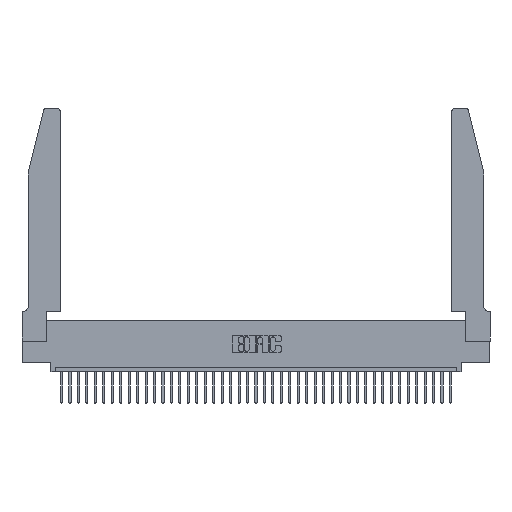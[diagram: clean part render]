
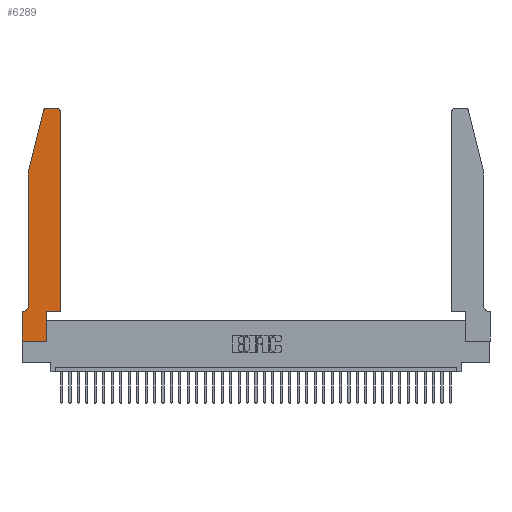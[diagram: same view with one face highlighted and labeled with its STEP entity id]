
A CAD part, top view. The second image highlights one B-rep face of the part: STEP entity #6289.
In plain terms, the highlighted planar face has unit normal (0, 0, 1).
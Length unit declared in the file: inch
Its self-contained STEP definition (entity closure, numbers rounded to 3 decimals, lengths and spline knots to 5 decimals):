
#177 = VECTOR ( 'NONE', #949, 39.37008 ) ;
#435 = CARTESIAN_POINT ( 'NONE',  ( 0.4205, 2.72, 0.37 ) ) ;
#949 = DIRECTION ( 'NONE',  ( -0.239, -0.971, 0. ) ) ;
#974 = CARTESIAN_POINT ( 'NONE',  ( 0.4505, 2.72, 0.37 ) ) ;
#1159 = VERTEX_POINT ( 'NONE', #22262 ) ;
#2561 = DIRECTION ( 'NONE',  ( -1., 0., 0. ) ) ;
#2755 = VERTEX_POINT ( 'NONE', #37232 ) ;
#3461 = DIRECTION ( 'NONE',  ( 1., 0., 0. ) ) ;
#4539 = AXIS2_PLACEMENT_3D ( 'NONE', #435, #18755, #3461 ) ;
#4997 = CARTESIAN_POINT ( 'NONE',  ( 0.0755, 2., 0.37 ) ) ;
#5003 = DIRECTION ( 'NONE',  ( 0., -1., 0. ) ) ;
#5371 = VERTEX_POINT ( 'NONE', #32633 ) ;
#5755 = ORIENTED_EDGE ( 'NONE', *, *, #23626, .T. ) ;
#6289 = ADVANCED_FACE ( 'NONE', ( #22251 ), #21122, .T. ) ;
#6807 = EDGE_CURVE ( 'NONE', #11209, #15292, #15464, .T. ) ;
#7222 = CARTESIAN_POINT ( 'NONE',  ( 0.4505, 0.35, 0.37 ) ) ;
#7364 = DIRECTION ( 'NONE',  ( 0., 1., 0. ) ) ;
#7656 = EDGE_CURVE ( 'NONE', #9898, #8906, #37901, .T. ) ;
#8488 = AXIS2_PLACEMENT_3D ( 'NONE', #20521, #39113, #36181 ) ;
#8906 = VERTEX_POINT ( 'NONE', #974 ) ;
#8969 = LINE ( 'NONE', #7222, #15138 ) ;
#9872 = CARTESIAN_POINT ( 'NONE',  ( 0.2865, 0.35, 0.37 ) ) ;
#9898 = VERTEX_POINT ( 'NONE', #19465 ) ;
#10765 = VECTOR ( 'NONE', #7364, 39.37008 ) ;
#11044 = CARTESIAN_POINT ( 'NONE',  ( 0., 0., 0.37 ) ) ;
#11209 = VERTEX_POINT ( 'NONE', #37685 ) ;
#11580 = ORIENTED_EDGE ( 'NONE', *, *, #13418, .T. ) ;
#11906 = VERTEX_POINT ( 'NONE', #21296 ) ;
#12608 = ORIENTED_EDGE ( 'NONE', *, *, #18195, .T. ) ;
#13418 = EDGE_CURVE ( 'NONE', #15748, #2755, #25089, .T. ) ;
#13810 = VERTEX_POINT ( 'NONE', #26644 ) ;
#13892 = DIRECTION ( 'NONE',  ( 0., 0., 1. ) ) ;
#14396 = DIRECTION ( 'NONE',  ( 1., 0., 0. ) ) ;
#14996 = LINE ( 'NONE', #34381, #177 ) ;
#15138 = VECTOR ( 'NONE', #14396, 39.37008 ) ;
#15172 = AXIS2_PLACEMENT_3D ( 'NONE', #37319, #24771, #15403 ) ;
#15292 = VERTEX_POINT ( 'NONE', #35835 ) ;
#15332 = CIRCLE ( 'NONE', #4539, 0.03 ) ;
#15403 = DIRECTION ( 'NONE',  ( 1., 0., 0. ) ) ;
#15464 = LINE ( 'NONE', #4997, #24592 ) ;
#15748 = VERTEX_POINT ( 'NONE', #31536 ) ;
#16007 = LINE ( 'NONE', #39061, #39537 ) ;
#16443 = LINE ( 'NONE', #9872, #10765 ) ;
#16594 = CARTESIAN_POINT ( 'NONE',  ( 0.284, 2.72, 0.37 ) ) ;
#17100 = EDGE_CURVE ( 'NONE', #2755, #13810, #16007, .T. ) ;
#17483 = VECTOR ( 'NONE', #32463, 39.37008 ) ;
#17523 = DIRECTION ( 'NONE',  ( 1., 0., 0. ) ) ;
#18100 = VERTEX_POINT ( 'NONE', #32592 ) ;
#18192 = ORIENTED_EDGE ( 'NONE', *, *, #6807, .T. ) ;
#18195 = EDGE_CURVE ( 'NONE', #11906, #5371, #33679, .T. ) ;
#18252 = EDGE_CURVE ( 'NONE', #5371, #1159, #33200, .T. ) ;
#18546 = VERTEX_POINT ( 'NONE', #32079 ) ;
#18755 = DIRECTION ( 'NONE',  ( 0., 0., 1. ) ) ;
#19384 = LINE ( 'NONE', #25616, #34694 ) ;
#19465 = CARTESIAN_POINT ( 'NONE',  ( 0.4505, 0.35, 0.37 ) ) ;
#20351 = EDGE_CURVE ( 'NONE', #15292, #18546, #33997, .T. ) ;
#20521 = CARTESIAN_POINT ( 'NONE',  ( 0.0055, 0.42, 0.37 ) ) ;
#21122 = PLANE ( 'NONE',  #15172 ) ;
#21296 = CARTESIAN_POINT ( 'NONE',  ( 0.4205, 2.75, 0.37 ) ) ;
#22251 = FACE_OUTER_BOUND ( 'NONE', #27820, .T. ) ;
#22262 = CARTESIAN_POINT ( 'NONE',  ( 0.25487, 2.72718, 0.37 ) ) ;
#22416 = EDGE_CURVE ( 'NONE', #18100, #9898, #8969, .T. ) ;
#23135 = ORIENTED_EDGE ( 'NONE', *, *, #23229, .T. ) ;
#23229 = EDGE_CURVE ( 'NONE', #18546, #15748, #19384, .T. ) ;
#23626 = EDGE_CURVE ( 'NONE', #13810, #18100, #16443, .T. ) ;
#24422 = ORIENTED_EDGE ( 'NONE', *, *, #18252, .T. ) ;
#24592 = VECTOR ( 'NONE', #5003, 39.37008 ) ;
#24771 = DIRECTION ( 'NONE',  ( 0., 0., 1. ) ) ;
#24855 = DIRECTION ( 'NONE',  ( 0., 1., 0. ) ) ;
#24994 = VECTOR ( 'NONE', #2561, 39.37008 ) ;
#25022 = ORIENTED_EDGE ( 'NONE', *, *, #17100, .T. ) ;
#25089 = LINE ( 'NONE', #11044, #17483 ) ;
#25457 = VECTOR ( 'NONE', #24855, 39.37008 ) ;
#25616 = CARTESIAN_POINT ( 'NONE',  ( 0.0755, 0.35, 0.37 ) ) ;
#25671 = DIRECTION ( 'NONE',  ( 1., 0., 0. ) ) ;
#25927 = ORIENTED_EDGE ( 'NONE', *, *, #20351, .T. ) ;
#25966 = CARTESIAN_POINT ( 'NONE',  ( 0.4505, 0.35, 0.37 ) ) ;
#26644 = CARTESIAN_POINT ( 'NONE',  ( 0.2865, 0., 0.37 ) ) ;
#27820 = EDGE_LOOP ( 'NONE', ( #12608, #24422, #38621, #18192, #25927, #23135, #11580, #25022, #5755, #35862, #31371, #34451 ) ) ;
#29533 = AXIS2_PLACEMENT_3D ( 'NONE', #16594, #13892, #25671 ) ;
#29898 = CARTESIAN_POINT ( 'NONE',  ( 0.2605, 2.75, 0.37 ) ) ;
#30116 = EDGE_CURVE ( 'NONE', #8906, #11906, #15332, .T. ) ;
#31371 = ORIENTED_EDGE ( 'NONE', *, *, #7656, .T. ) ;
#31536 = CARTESIAN_POINT ( 'NONE',  ( 0., 0.35, 0.37 ) ) ;
#32079 = CARTESIAN_POINT ( 'NONE',  ( 0.0055, 0.35, 0.37 ) ) ;
#32463 = DIRECTION ( 'NONE',  ( 0., -1., 0. ) ) ;
#32592 = CARTESIAN_POINT ( 'NONE',  ( 0.2865, 0.35, 0.37 ) ) ;
#32633 = CARTESIAN_POINT ( 'NONE',  ( 0.284, 2.75, 0.37 ) ) ;
#33200 = CIRCLE ( 'NONE', #29533, 0.03 ) ;
#33679 = LINE ( 'NONE', #29898, #24994 ) ;
#33997 = CIRCLE ( 'NONE', #8488, 0.07 ) ;
#34381 = CARTESIAN_POINT ( 'NONE',  ( 0.0755, 2., 0.37 ) ) ;
#34451 = ORIENTED_EDGE ( 'NONE', *, *, #30116, .T. ) ;
#34694 = VECTOR ( 'NONE', #38193, 39.37008 ) ;
#35835 = CARTESIAN_POINT ( 'NONE',  ( 0.0755, 0.42, 0.37 ) ) ;
#35862 = ORIENTED_EDGE ( 'NONE', *, *, #22416, .T. ) ;
#36181 = DIRECTION ( 'NONE',  ( -1., 0., 0. ) ) ;
#37211 = EDGE_CURVE ( 'NONE', #1159, #11209, #14996, .T. ) ;
#37232 = CARTESIAN_POINT ( 'NONE',  ( 0., 0., 0.37 ) ) ;
#37319 = CARTESIAN_POINT ( 'NONE',  ( 0., 0.35, 0.37 ) ) ;
#37685 = CARTESIAN_POINT ( 'NONE',  ( 0.0755, 2., 0.37 ) ) ;
#37901 = LINE ( 'NONE', #25966, #25457 ) ;
#38193 = DIRECTION ( 'NONE',  ( -1., 0., 0. ) ) ;
#38621 = ORIENTED_EDGE ( 'NONE', *, *, #37211, .T. ) ;
#39061 = CARTESIAN_POINT ( 'NONE',  ( 0., 0., 0.37 ) ) ;
#39113 = DIRECTION ( 'NONE',  ( 0., 0., -1. ) ) ;
#39537 = VECTOR ( 'NONE', #17523, 39.37008 ) ;
